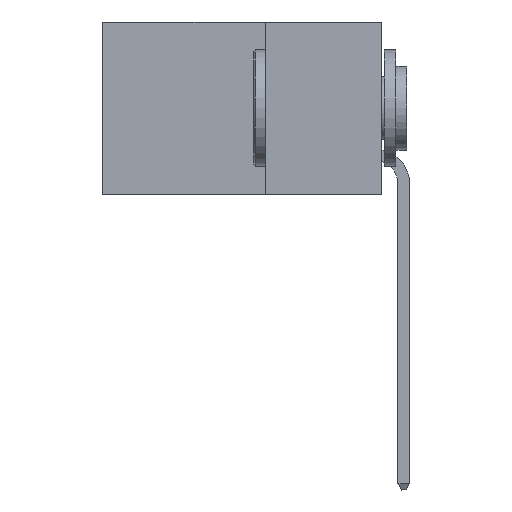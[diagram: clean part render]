
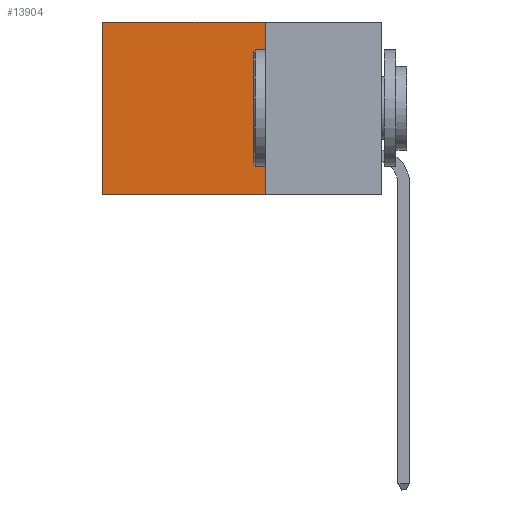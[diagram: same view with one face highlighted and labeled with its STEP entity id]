
A CAD part, left-side view. The second image highlights one B-rep face of the part: STEP entity #13904.
In plain terms, the highlighted planar face has unit normal (-1, 0, 0).
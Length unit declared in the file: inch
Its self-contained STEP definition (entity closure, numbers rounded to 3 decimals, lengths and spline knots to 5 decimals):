
#33 = CARTESIAN_POINT ( 'NONE',  ( 0.2875, 0.6, -0.37 ) ) ;
#393 = CARTESIAN_POINT ( 'NONE',  ( 0.2875, 0.25, -0.37 ) ) ;
#581 = LINE ( 'NONE', #12089, #18405 ) ;
#650 = CARTESIAN_POINT ( 'NONE',  ( 0.2875, 0.25, 0. ) ) ;
#1891 = AXIS2_PLACEMENT_3D ( 'NONE', #650, #18087, #16700 ) ;
#2154 = VERTEX_POINT ( 'NONE', #13722 ) ;
#4856 = EDGE_CURVE ( 'NONE', #18986, #19472, #17431, .T. ) ;
#5428 = EDGE_CURVE ( 'NONE', #2154, #19472, #14655, .T. ) ;
#6336 = LINE ( 'NONE', #20985, #7152 ) ;
#6542 = VERTEX_POINT ( 'NONE', #7870 ) ;
#7152 = VECTOR ( 'NONE', #15729, 39.37008 ) ;
#7385 = VECTOR ( 'NONE', #16295, 39.37008 ) ;
#7870 = CARTESIAN_POINT ( 'NONE',  ( 0.2875, 0.25, 0. ) ) ;
#8421 = EDGE_CURVE ( 'NONE', #6542, #2154, #6336, .T. ) ;
#8899 = FACE_OUTER_BOUND ( 'NONE', #13527, .T. ) ;
#9943 = DIRECTION ( 'NONE',  ( 0., 1., 0. ) ) ;
#11732 = EDGE_CURVE ( 'NONE', #6542, #18986, #581, .T. ) ;
#12089 = CARTESIAN_POINT ( 'NONE',  ( 0.2875, 0.25, 0. ) ) ;
#12776 = CARTESIAN_POINT ( 'NONE',  ( 0.2875, 0.6, 0. ) ) ;
#13527 = EDGE_LOOP ( 'NONE', ( #20117, #22529, #16763, #17833 ) ) ;
#13722 = CARTESIAN_POINT ( 'NONE',  ( 0.2875, 0.25, -0.37 ) ) ;
#13904 = ADVANCED_FACE ( 'NONE', ( #8899 ), #21975, .F. ) ;
#14655 = LINE ( 'NONE', #393, #7385 ) ;
#15729 = DIRECTION ( 'NONE',  ( 0., 0., -1. ) ) ;
#16295 = DIRECTION ( 'NONE',  ( 0., 1., 0. ) ) ;
#16700 = DIRECTION ( 'NONE',  ( 0., 0., -1. ) ) ;
#16763 = ORIENTED_EDGE ( 'NONE', *, *, #8421, .F. ) ;
#16822 = DIRECTION ( 'NONE',  ( 0., 0., -1. ) ) ;
#17431 = LINE ( 'NONE', #20149, #19375 ) ;
#17833 = ORIENTED_EDGE ( 'NONE', *, *, #11732, .T. ) ;
#18087 = DIRECTION ( 'NONE',  ( 1., 0., 0. ) ) ;
#18405 = VECTOR ( 'NONE', #9943, 39.37008 ) ;
#18986 = VERTEX_POINT ( 'NONE', #12776 ) ;
#19375 = VECTOR ( 'NONE', #16822, 39.37008 ) ;
#19472 = VERTEX_POINT ( 'NONE', #33 ) ;
#20117 = ORIENTED_EDGE ( 'NONE', *, *, #4856, .T. ) ;
#20149 = CARTESIAN_POINT ( 'NONE',  ( 0.2875, 0.6, 0. ) ) ;
#20985 = CARTESIAN_POINT ( 'NONE',  ( 0.2875, 0.25, 0. ) ) ;
#21975 = PLANE ( 'NONE',  #1891 ) ;
#22529 = ORIENTED_EDGE ( 'NONE', *, *, #5428, .F. ) ;
